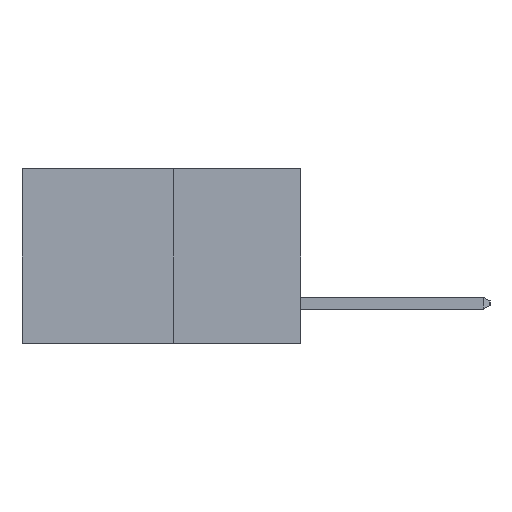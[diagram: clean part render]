
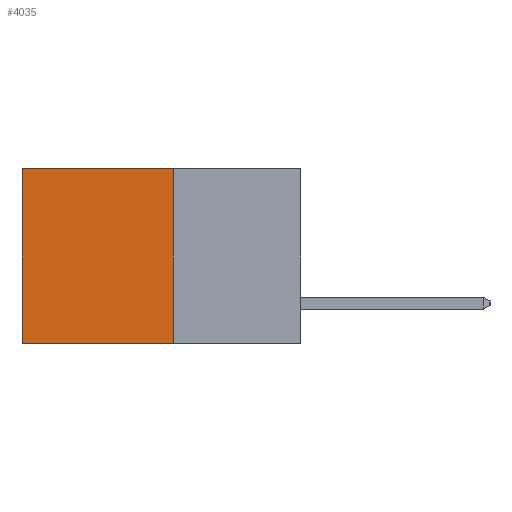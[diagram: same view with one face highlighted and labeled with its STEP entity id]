
A CAD part, left-side view. The second image highlights one B-rep face of the part: STEP entity #4035.
In plain terms, the highlighted planar face has unit normal (-1, 0, 0).
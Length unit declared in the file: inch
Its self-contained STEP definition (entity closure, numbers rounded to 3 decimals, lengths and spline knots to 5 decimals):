
#6 = EDGE_LOOP ( 'NONE', ( #349, #16762, #13320, #17642 ) ) ;
#349 = ORIENTED_EDGE ( 'NONE', *, *, #5040, .T. ) ;
#613 = DIRECTION ( 'NONE',  ( 0., 1., 0. ) ) ;
#1180 = PLANE ( 'NONE',  #13997 ) ;
#1330 = LINE ( 'NONE', #19026, #16791 ) ;
#1621 = VERTEX_POINT ( 'NONE', #10077 ) ;
#2536 = CARTESIAN_POINT ( 'NONE',  ( 0.277, 0.27, -0.37 ) ) ;
#3315 = VERTEX_POINT ( 'NONE', #2536 ) ;
#4035 = ADVANCED_FACE ( 'NONE', ( #6922 ), #1180, .F. ) ;
#4274 = LINE ( 'NONE', #5137, #15687 ) ;
#5040 = EDGE_CURVE ( 'NONE', #10396, #1621, #12088, .T. ) ;
#5137 = CARTESIAN_POINT ( 'NONE',  ( 0.277, 0.27, 0. ) ) ;
#6257 = EDGE_CURVE ( 'NONE', #3315, #1621, #10860, .T. ) ;
#6381 = VECTOR ( 'NONE', #15797, 39.37008 ) ;
#6922 = FACE_OUTER_BOUND ( 'NONE', #6, .T. ) ;
#8207 = DIRECTION ( 'NONE',  ( 0., 0., -1. ) ) ;
#9400 = DIRECTION ( 'NONE',  ( 1., 0., 0. ) ) ;
#10077 = CARTESIAN_POINT ( 'NONE',  ( 0.277, 0.59, -0.37 ) ) ;
#10219 = CARTESIAN_POINT ( 'NONE',  ( 0.277, 0.27, -0.37 ) ) ;
#10396 = VERTEX_POINT ( 'NONE', #12492 ) ;
#10860 = LINE ( 'NONE', #10219, #6381 ) ;
#10951 = CARTESIAN_POINT ( 'NONE',  ( 0.277, 0.27, -0.37 ) ) ;
#11647 = CARTESIAN_POINT ( 'NONE',  ( 0.277, 0.27, 0. ) ) ;
#11744 = DIRECTION ( 'NONE',  ( 0., 0., -1. ) ) ;
#12039 = EDGE_CURVE ( 'NONE', #15034, #10396, #4274, .T. ) ;
#12088 = LINE ( 'NONE', #17678, #15518 ) ;
#12492 = CARTESIAN_POINT ( 'NONE',  ( 0.277, 0.59, 0. ) ) ;
#13320 = ORIENTED_EDGE ( 'NONE', *, *, #13538, .F. ) ;
#13538 = EDGE_CURVE ( 'NONE', #15034, #3315, #1330, .T. ) ;
#13997 = AXIS2_PLACEMENT_3D ( 'NONE', #10951, #9400, #14264 ) ;
#14264 = DIRECTION ( 'NONE',  ( 0., 0., -1. ) ) ;
#15034 = VERTEX_POINT ( 'NONE', #11647 ) ;
#15518 = VECTOR ( 'NONE', #8207, 39.37008 ) ;
#15687 = VECTOR ( 'NONE', #613, 39.37008 ) ;
#15797 = DIRECTION ( 'NONE',  ( 0., 1., 0. ) ) ;
#16762 = ORIENTED_EDGE ( 'NONE', *, *, #6257, .F. ) ;
#16791 = VECTOR ( 'NONE', #11744, 39.37008 ) ;
#17642 = ORIENTED_EDGE ( 'NONE', *, *, #12039, .T. ) ;
#17678 = CARTESIAN_POINT ( 'NONE',  ( 0.277, 0.59, -0.37 ) ) ;
#19026 = CARTESIAN_POINT ( 'NONE',  ( 0.277, 0.27, -0.37 ) ) ;
